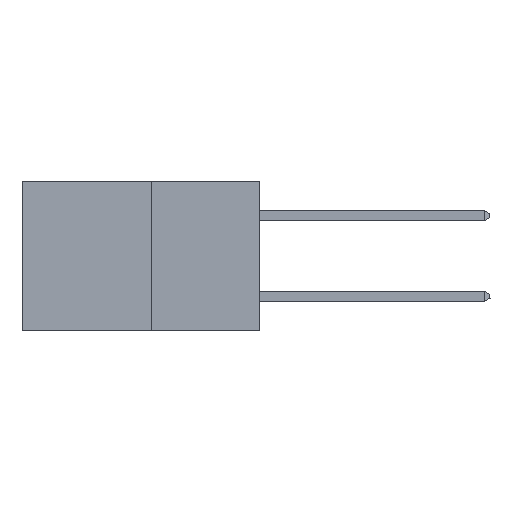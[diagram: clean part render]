
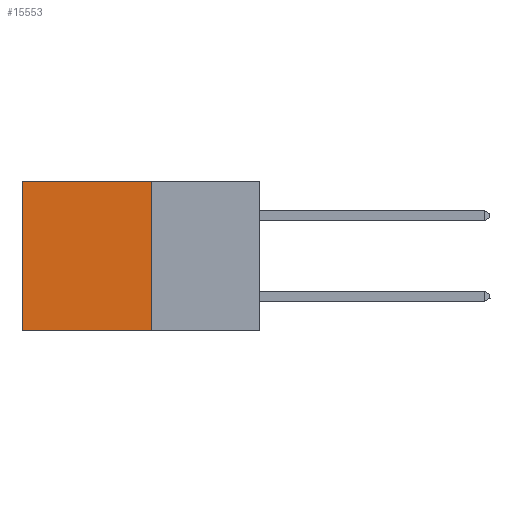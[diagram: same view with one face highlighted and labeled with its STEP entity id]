
A CAD part, left-side view. The second image highlights one B-rep face of the part: STEP entity #15553.
In plain terms, the highlighted planar face has unit normal (-1, 0, 0).
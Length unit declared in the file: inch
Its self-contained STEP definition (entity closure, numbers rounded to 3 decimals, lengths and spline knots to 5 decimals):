
#500 = CARTESIAN_POINT ( 'NONE',  ( 0.277, 0.27, 0. ) ) ;
#1309 = CARTESIAN_POINT ( 'NONE',  ( 0.277, 0.27, -0.37 ) ) ;
#1440 = PLANE ( 'NONE',  #4652 ) ;
#1548 = LINE ( 'NONE', #1309, #5400 ) ;
#2178 = LINE ( 'NONE', #17932, #18811 ) ;
#2227 = VERTEX_POINT ( 'NONE', #4800 ) ;
#2896 = VECTOR ( 'NONE', #17740, 39.37008 ) ;
#3333 = DIRECTION ( 'NONE',  ( 0., 0., -1. ) ) ;
#4652 = AXIS2_PLACEMENT_3D ( 'NONE', #9015, #14733, #3333 ) ;
#4800 = CARTESIAN_POINT ( 'NONE',  ( 0.277, 0.59, -0.37 ) ) ;
#5254 = EDGE_CURVE ( 'NONE', #14885, #2227, #2178, .T. ) ;
#5400 = VECTOR ( 'NONE', #20242, 39.37008 ) ;
#5562 = FACE_OUTER_BOUND ( 'NONE', #21365, .T. ) ;
#6345 = CARTESIAN_POINT ( 'NONE',  ( 0.277, 0.59, -0.37 ) ) ;
#7071 = ORIENTED_EDGE ( 'NONE', *, *, #23555, .F. ) ;
#8677 = EDGE_CURVE ( 'NONE', #16636, #11944, #11421, .T. ) ;
#9015 = CARTESIAN_POINT ( 'NONE',  ( 0.277, 0.27, -0.37 ) ) ;
#9732 = ORIENTED_EDGE ( 'NONE', *, *, #5254, .F. ) ;
#11421 = LINE ( 'NONE', #15663, #20817 ) ;
#11944 = VERTEX_POINT ( 'NONE', #21391 ) ;
#12487 = EDGE_CURVE ( 'NONE', #11944, #2227, #18063, .T. ) ;
#12858 = ORIENTED_EDGE ( 'NONE', *, *, #8677, .T. ) ;
#14733 = DIRECTION ( 'NONE',  ( 1., 0., 0. ) ) ;
#14885 = VERTEX_POINT ( 'NONE', #21781 ) ;
#15553 = ADVANCED_FACE ( 'NONE', ( #5562 ), #1440, .F. ) ;
#15663 = CARTESIAN_POINT ( 'NONE',  ( 0.277, 0.27, 0. ) ) ;
#16636 = VERTEX_POINT ( 'NONE', #500 ) ;
#17218 = DIRECTION ( 'NONE',  ( 0., 1., 0. ) ) ;
#17576 = DIRECTION ( 'NONE',  ( 0., 1., 0. ) ) ;
#17740 = DIRECTION ( 'NONE',  ( 0., 0., -1. ) ) ;
#17932 = CARTESIAN_POINT ( 'NONE',  ( 0.277, 0.27, -0.37 ) ) ;
#18063 = LINE ( 'NONE', #6345, #2896 ) ;
#18811 = VECTOR ( 'NONE', #17218, 39.37008 ) ;
#20231 = ORIENTED_EDGE ( 'NONE', *, *, #12487, .T. ) ;
#20242 = DIRECTION ( 'NONE',  ( 0., 0., -1. ) ) ;
#20817 = VECTOR ( 'NONE', #17576, 39.37008 ) ;
#21365 = EDGE_LOOP ( 'NONE', ( #20231, #9732, #7071, #12858 ) ) ;
#21391 = CARTESIAN_POINT ( 'NONE',  ( 0.277, 0.59, 0. ) ) ;
#21781 = CARTESIAN_POINT ( 'NONE',  ( 0.277, 0.27, -0.37 ) ) ;
#23555 = EDGE_CURVE ( 'NONE', #16636, #14885, #1548, .T. ) ;
